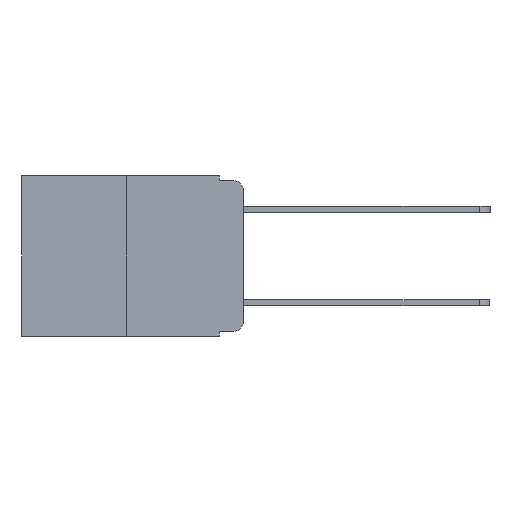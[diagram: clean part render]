
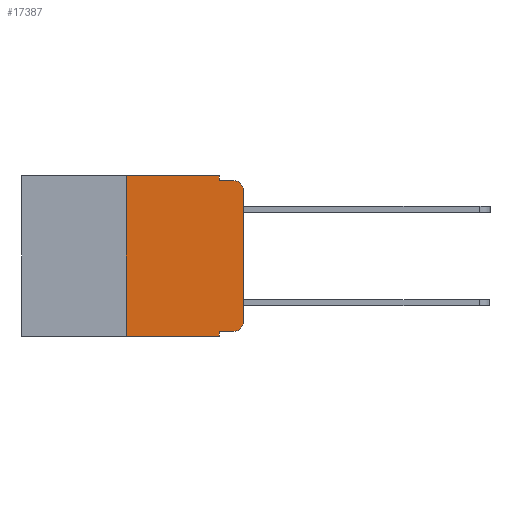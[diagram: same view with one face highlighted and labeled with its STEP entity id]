
A CAD part, left-side view. The second image highlights one B-rep face of the part: STEP entity #17387.
In plain terms, the highlighted planar face has unit normal (-1, 0, 0).
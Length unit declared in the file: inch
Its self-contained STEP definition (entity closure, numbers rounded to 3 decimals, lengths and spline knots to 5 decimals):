
#745 = CARTESIAN_POINT ( 'NONE',  ( 0., 0.02, -0.01 ) ) ;
#801 = VERTEX_POINT ( 'NONE', #16017 ) ;
#1287 = AXIS2_PLACEMENT_3D ( 'NONE', #2160, #2082, #2004 ) ;
#1541 = VERTEX_POINT ( 'NONE', #745 ) ;
#1620 = EDGE_CURVE ( 'NONE', #4217, #1541, #23147, .T. ) ;
#1719 = CARTESIAN_POINT ( 'NONE',  ( 0., 0.25, 0. ) ) ;
#1917 = ORIENTED_EDGE ( 'NONE', *, *, #23168, .T. ) ;
#1958 = VECTOR ( 'NONE', #4683, 39.37008 ) ;
#2004 = DIRECTION ( 'NONE',  ( 0., 0., -1. ) ) ;
#2082 = DIRECTION ( 'NONE',  ( -1., 0., 0. ) ) ;
#2160 = CARTESIAN_POINT ( 'NONE',  ( 0., 0.02, -0.03 ) ) ;
#2245 = CARTESIAN_POINT ( 'NONE',  ( 0., 0., -0.313 ) ) ;
#2289 = CARTESIAN_POINT ( 'NONE',  ( 0., 0.02, -0.333 ) ) ;
#2641 = EDGE_CURVE ( 'NONE', #22889, #12684, #5485, .T. ) ;
#2697 = VECTOR ( 'NONE', #17318, 39.37008 ) ;
#2989 = CARTESIAN_POINT ( 'NONE',  ( 0., 0.051, -0.333 ) ) ;
#3029 = LINE ( 'NONE', #2989, #23513 ) ;
#3768 = CARTESIAN_POINT ( 'NONE',  ( 0., 0.25, 0. ) ) ;
#4217 = VERTEX_POINT ( 'NONE', #16820 ) ;
#4237 = CARTESIAN_POINT ( 'NONE',  ( 0., 0.473, 0. ) ) ;
#4349 = EDGE_CURVE ( 'NONE', #19079, #1541, #16577, .T. ) ;
#4683 = DIRECTION ( 'NONE',  ( 0., -1., 0. ) ) ;
#5406 = CARTESIAN_POINT ( 'NONE',  ( 0., 0.473, 0. ) ) ;
#5485 = CIRCLE ( 'NONE', #25551, 0.02 ) ;
#5662 = VERTEX_POINT ( 'NONE', #15980 ) ;
#6267 = DIRECTION ( 'NONE',  ( 1., 0., 0. ) ) ;
#7084 = CARTESIAN_POINT ( 'NONE',  ( 0., 0.02, -0.313 ) ) ;
#7125 = DIRECTION ( 'NONE',  ( -1., 0., 0. ) ) ;
#7586 = DIRECTION ( 'NONE',  ( 0., 0., -1. ) ) ;
#7997 = EDGE_CURVE ( 'NONE', #11267, #22889, #3029, .T. ) ;
#8905 = ORIENTED_EDGE ( 'NONE', *, *, #4349, .T. ) ;
#8930 = DIRECTION ( 'NONE',  ( 0., 0., 1. ) ) ;
#10050 = ORIENTED_EDGE ( 'NONE', *, *, #15458, .F. ) ;
#11126 = VECTOR ( 'NONE', #8930, 39.37008 ) ;
#11211 = DIRECTION ( 'NONE',  ( 0., -1., 0. ) ) ;
#11267 = VERTEX_POINT ( 'NONE', #20351 ) ;
#11523 = DIRECTION ( 'NONE',  ( 0., 0., -1. ) ) ;
#12352 = EDGE_CURVE ( 'NONE', #12684, #19079, #17035, .T. ) ;
#12431 = ORIENTED_EDGE ( 'NONE', *, *, #24746, .F. ) ;
#12634 = VECTOR ( 'NONE', #7586, 39.37008 ) ;
#12684 = VERTEX_POINT ( 'NONE', #2245 ) ;
#13262 = LINE ( 'NONE', #19580, #12634 ) ;
#13279 = LINE ( 'NONE', #20140, #23201 ) ;
#13296 = LINE ( 'NONE', #5406, #2697 ) ;
#14899 = VERTEX_POINT ( 'NONE', #21483 ) ;
#15127 = CARTESIAN_POINT ( 'NONE',  ( 0., 0.473, -0.343 ) ) ;
#15458 = EDGE_CURVE ( 'NONE', #21004, #14899, #13296, .T. ) ;
#15980 = CARTESIAN_POINT ( 'NONE',  ( 0., 0.051, -0.343 ) ) ;
#16017 = CARTESIAN_POINT ( 'NONE',  ( 0., 0.25, -0.343 ) ) ;
#16091 = ORIENTED_EDGE ( 'NONE', *, *, #7997, .T. ) ;
#16166 = PLANE ( 'NONE',  #23072 ) ;
#16418 = ORIENTED_EDGE ( 'NONE', *, *, #2641, .T. ) ;
#16577 = CIRCLE ( 'NONE', #1287, 0.02 ) ;
#16820 = CARTESIAN_POINT ( 'NONE',  ( 0., 0.051, -0.01 ) ) ;
#16903 = DIRECTION ( 'NONE',  ( 0., -1., 0. ) ) ;
#17035 = LINE ( 'NONE', #20819, #11126 ) ;
#17318 = DIRECTION ( 'NONE',  ( 0., -1., 0. ) ) ;
#17387 = ADVANCED_FACE ( 'NONE', ( #19966 ), #16166, .F. ) ;
#19079 = VERTEX_POINT ( 'NONE', #23002 ) ;
#19195 = VECTOR ( 'NONE', #23616, 39.37008 ) ;
#19233 = ORIENTED_EDGE ( 'NONE', *, *, #1620, .F. ) ;
#19580 = CARTESIAN_POINT ( 'NONE',  ( 0., 0.051, 0. ) ) ;
#19966 = FACE_OUTER_BOUND ( 'NONE', #25799, .T. ) ;
#20140 = CARTESIAN_POINT ( 'NONE',  ( 0., 0.051, 0. ) ) ;
#20153 = DIRECTION ( 'NONE',  ( 0., 0., -1. ) ) ;
#20351 = CARTESIAN_POINT ( 'NONE',  ( 0., 0.051, -0.333 ) ) ;
#20659 = VECTOR ( 'NONE', #11211, 39.37008 ) ;
#20819 = CARTESIAN_POINT ( 'NONE',  ( 0., 0., 0. ) ) ;
#21004 = VERTEX_POINT ( 'NONE', #1719 ) ;
#21483 = CARTESIAN_POINT ( 'NONE',  ( 0., 0.051, 0. ) ) ;
#21849 = ORIENTED_EDGE ( 'NONE', *, *, #22133, .F. ) ;
#22133 = EDGE_CURVE ( 'NONE', #801, #21004, #24390, .T. ) ;
#22629 = EDGE_CURVE ( 'NONE', #11267, #5662, #13262, .T. ) ;
#22889 = VERTEX_POINT ( 'NONE', #2289 ) ;
#23002 = CARTESIAN_POINT ( 'NONE',  ( 0., 0., -0.03 ) ) ;
#23072 = AXIS2_PLACEMENT_3D ( 'NONE', #4237, #6267, #20153 ) ;
#23147 = LINE ( 'NONE', #23942, #1958 ) ;
#23168 = EDGE_CURVE ( 'NONE', #801, #5662, #25830, .T. ) ;
#23201 = VECTOR ( 'NONE', #24057, 39.37008 ) ;
#23513 = VECTOR ( 'NONE', #16903, 39.37008 ) ;
#23616 = DIRECTION ( 'NONE',  ( 0., 0., 1. ) ) ;
#23942 = CARTESIAN_POINT ( 'NONE',  ( 0., 0.051, -0.01 ) ) ;
#24057 = DIRECTION ( 'NONE',  ( 0., 0., -1. ) ) ;
#24283 = ORIENTED_EDGE ( 'NONE', *, *, #22629, .F. ) ;
#24354 = ORIENTED_EDGE ( 'NONE', *, *, #12352, .T. ) ;
#24390 = LINE ( 'NONE', #3768, #19195 ) ;
#24746 = EDGE_CURVE ( 'NONE', #14899, #4217, #13279, .T. ) ;
#25551 = AXIS2_PLACEMENT_3D ( 'NONE', #7084, #7125, #11523 ) ;
#25799 = EDGE_LOOP ( 'NONE', ( #24354, #8905, #19233, #12431, #10050, #21849, #1917, #24283, #16091, #16418 ) ) ;
#25830 = LINE ( 'NONE', #15127, #20659 ) ;
